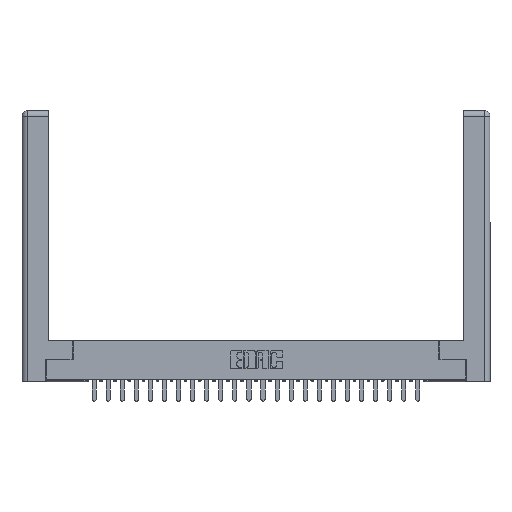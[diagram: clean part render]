
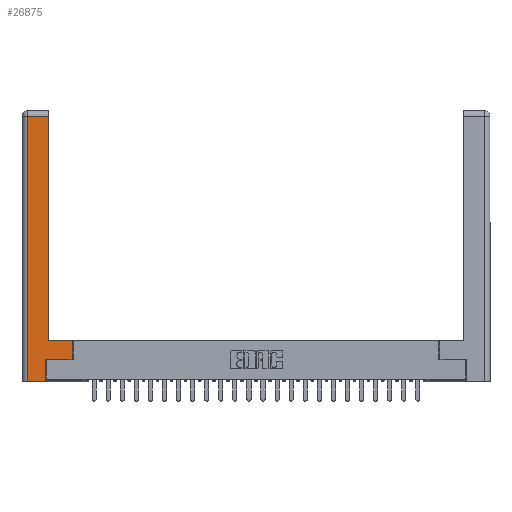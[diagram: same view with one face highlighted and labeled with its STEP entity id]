
A CAD part, top view. The second image highlights one B-rep face of the part: STEP entity #26875.
In plain terms, the highlighted planar face has unit normal (0, 0, 1).
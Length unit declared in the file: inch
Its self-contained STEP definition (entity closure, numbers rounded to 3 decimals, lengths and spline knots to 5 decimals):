
#244 = VECTOR ( 'NONE', #6584, 39.37008 ) ;
#1104 = CARTESIAN_POINT ( 'NONE',  ( 0.265, 0.245, 0. ) ) ;
#1761 = DIRECTION ( 'NONE',  ( 1., 0., 0. ) ) ;
#1874 = DIRECTION ( 'NONE',  ( -1., 0., 0. ) ) ;
#1884 = ORIENTED_EDGE ( 'NONE', *, *, #8562, .T. ) ;
#2675 = CARTESIAN_POINT ( 'NONE',  ( 0.0615, 0., 0. ) ) ;
#3202 = DIRECTION ( 'NONE',  ( 0., 1., 0. ) ) ;
#3959 = CARTESIAN_POINT ( 'NONE',  ( 0.565, 0.245, 0. ) ) ;
#4890 = VERTEX_POINT ( 'NONE', #14728 ) ;
#4986 = VERTEX_POINT ( 'NONE', #19668 ) ;
#5366 = DIRECTION ( 'NONE',  ( -1., 0., 0. ) ) ;
#6485 = VERTEX_POINT ( 'NONE', #1104 ) ;
#6584 = DIRECTION ( 'NONE',  ( 0., 1., 0. ) ) ;
#6752 = LINE ( 'NONE', #21202, #244 ) ;
#7058 = ORIENTED_EDGE ( 'NONE', *, *, #19336, .T. ) ;
#7447 = CARTESIAN_POINT ( 'NONE',  ( 0.295, 0.45, 0. ) ) ;
#7497 = AXIS2_PLACEMENT_3D ( 'NONE', #8251, #14554, #1874 ) ;
#7553 = CARTESIAN_POINT ( 'NONE',  ( 0.0615, 0., 0. ) ) ;
#8178 = DIRECTION ( 'NONE',  ( -1., 0., 0. ) ) ;
#8188 = VERTEX_POINT ( 'NONE', #16981 ) ;
#8251 = CARTESIAN_POINT ( 'NONE',  ( 0., 0., 0. ) ) ;
#8457 = VERTEX_POINT ( 'NONE', #9813 ) ;
#8562 = EDGE_CURVE ( 'NONE', #8188, #4986, #11885, .T. ) ;
#9016 = VECTOR ( 'NONE', #19524, 39.37008 ) ;
#9092 = CARTESIAN_POINT ( 'NONE',  ( 0.265, 0., 0. ) ) ;
#9813 = CARTESIAN_POINT ( 'NONE',  ( 0.565, 0.45, 0. ) ) ;
#9859 = VERTEX_POINT ( 'NONE', #19952 ) ;
#9863 = EDGE_CURVE ( 'NONE', #9859, #6485, #27157, .T. ) ;
#10957 = ORIENTED_EDGE ( 'NONE', *, *, #9863, .T. ) ;
#11133 = LINE ( 'NONE', #9092, #26500 ) ;
#11825 = EDGE_CURVE ( 'NONE', #6485, #4890, #16316, .T. ) ;
#11885 = LINE ( 'NONE', #26964, #22396 ) ;
#12427 = PLANE ( 'NONE',  #7497 ) ;
#12448 = CARTESIAN_POINT ( 'NONE',  ( 0.295, 3., 0. ) ) ;
#12766 = ORIENTED_EDGE ( 'NONE', *, *, #11825, .T. ) ;
#14513 = FACE_OUTER_BOUND ( 'NONE', #17172, .T. ) ;
#14554 = DIRECTION ( 'NONE',  ( 0., 0., -1. ) ) ;
#14728 = CARTESIAN_POINT ( 'NONE',  ( 0.565, 0.245, 0. ) ) ;
#15018 = EDGE_CURVE ( 'NONE', #17921, #8188, #15166, .T. ) ;
#15166 = LINE ( 'NONE', #12448, #26268 ) ;
#15384 = VECTOR ( 'NONE', #5366, 39.37008 ) ;
#15756 = CARTESIAN_POINT ( 'NONE',  ( 0.265, 0.245, 0. ) ) ;
#16042 = LINE ( 'NONE', #26107, #15384 ) ;
#16316 = LINE ( 'NONE', #3959, #21880 ) ;
#16981 = CARTESIAN_POINT ( 'NONE',  ( 0.295, 2.94, 0. ) ) ;
#17172 = EDGE_LOOP ( 'NONE', ( #21489, #1884, #18872, #21322, #10957, #12766, #25339, #7058 ) ) ;
#17921 = VERTEX_POINT ( 'NONE', #7447 ) ;
#18872 = ORIENTED_EDGE ( 'NONE', *, *, #21560, .T. ) ;
#19336 = EDGE_CURVE ( 'NONE', #8457, #17921, #16042, .T. ) ;
#19524 = DIRECTION ( 'NONE',  ( 0., -1., 0. ) ) ;
#19668 = CARTESIAN_POINT ( 'NONE',  ( 0.0615, 2.94, 0. ) ) ;
#19952 = CARTESIAN_POINT ( 'NONE',  ( 0.265, 0., 0. ) ) ;
#20826 = LINE ( 'NONE', #2675, #9016 ) ;
#21202 = CARTESIAN_POINT ( 'NONE',  ( 0.565, 0.45, 0. ) ) ;
#21322 = ORIENTED_EDGE ( 'NONE', *, *, #24213, .T. ) ;
#21489 = ORIENTED_EDGE ( 'NONE', *, *, #15018, .T. ) ;
#21560 = EDGE_CURVE ( 'NONE', #4986, #24399, #20826, .T. ) ;
#21667 = VECTOR ( 'NONE', #3202, 39.37008 ) ;
#21741 = DIRECTION ( 'NONE',  ( 1., 0., 0. ) ) ;
#21880 = VECTOR ( 'NONE', #1761, 39.37008 ) ;
#22396 = VECTOR ( 'NONE', #8178, 39.37008 ) ;
#22906 = DIRECTION ( 'NONE',  ( 0., 1., 0. ) ) ;
#24213 = EDGE_CURVE ( 'NONE', #24399, #9859, #11133, .T. ) ;
#24399 = VERTEX_POINT ( 'NONE', #7553 ) ;
#25339 = ORIENTED_EDGE ( 'NONE', *, *, #25931, .T. ) ;
#25931 = EDGE_CURVE ( 'NONE', #4890, #8457, #6752, .T. ) ;
#26107 = CARTESIAN_POINT ( 'NONE',  ( 0.295, 0.45, 0. ) ) ;
#26268 = VECTOR ( 'NONE', #22906, 39.37008 ) ;
#26500 = VECTOR ( 'NONE', #21741, 39.37008 ) ;
#26875 = ADVANCED_FACE ( 'NONE', ( #14513 ), #12427, .F. ) ;
#26964 = CARTESIAN_POINT ( 'NONE',  ( 0.0615, 2.94, 0. ) ) ;
#27157 = LINE ( 'NONE', #15756, #21667 ) ;
